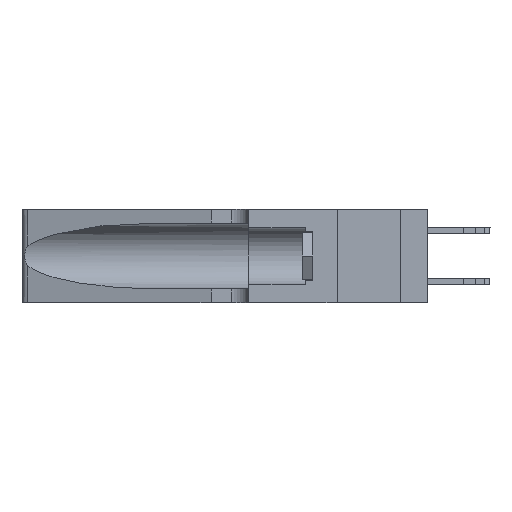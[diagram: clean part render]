
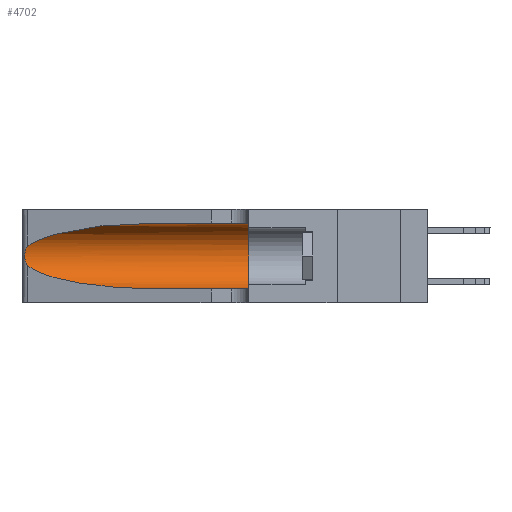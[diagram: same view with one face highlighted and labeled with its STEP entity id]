
A CAD part, left-side view. The second image highlights one B-rep face of the part: STEP entity #4702.
In plain terms, the highlighted cylindrical face has radius 3.308 mm (diameter 6.617 mm), a partial arc.
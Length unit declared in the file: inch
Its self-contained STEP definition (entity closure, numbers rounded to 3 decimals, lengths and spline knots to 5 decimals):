
#252 = CARTESIAN_POINT ( 'NONE',  ( 0.26018, 1.23835, 0.19895 ) ) ;
#362 = CARTESIAN_POINT ( 'NONE',  ( 0.25856, 1.23593, 0.16098 ) ) ;
#507 = CARTESIAN_POINT ( 'NONE',  ( 0.25487, 1.22718, 0.14631 ) ) ;
#692 = VERTEX_POINT ( 'NONE', #29806 ) ;
#1104 = ORIENTED_EDGE ( 'NONE', *, *, #36929, .T. ) ;
#3872 = CARTESIAN_POINT ( 'NONE',  ( 0.1305, 1.61858, 0.31525 ) ) ;
#4284 = CIRCLE ( 'NONE', #36613, 0.13025 ) ;
#4702 = ADVANCED_FACE ( 'NONE', ( #12334 ), #5035, .F. ) ;
#5035 = CYLINDRICAL_SURFACE ( 'NONE', #19683, 0.13025 ) ;
#5828 = DIRECTION ( 'NONE',  ( 0., -1., 0. ) ) ;
#6023 = CARTESIAN_POINT ( 'NONE',  ( 0.26075, 1.23896, 0.178 ) ) ;
#6257 = CARTESIAN_POINT ( 'NONE',  ( 0.25639, 1.23186, 0.15144 ) ) ;
#6469 = CARTESIAN_POINT ( 'NONE',  ( 0.1305, 1.61858, 0.05475 ) ) ;
#6514 = CARTESIAN_POINT ( 'NONE',  ( 0.25487, 1.22718, 0.22369 ) ) ;
#7052 =( BOUNDED_CURVE ( )  B_SPLINE_CURVE ( 3, ( #30509, #27434, #10241, #10376 ),
 .UNSPECIFIED., .F., .T. ) 
 B_SPLINE_CURVE_WITH_KNOTS ( ( 4, 4 ),
 ( 1.5708, 2.84003 ),
 .UNSPECIFIED. ) 
 CURVE ( )  GEOMETRIC_REPRESENTATION_ITEM ( )  RATIONAL_B_SPLINE_CURVE ( ( 1., 0.87, 0.87, 1. ) ) 
 REPRESENTATION_ITEM ( '' )  );
#7086 = ORIENTED_EDGE ( 'NONE', *, *, #24848, .T. ) ;
#7550 = CARTESIAN_POINT ( 'NONE',  ( 0.1305, 0.72297, 0.05475 ) ) ;
#9229 = CARTESIAN_POINT ( 'NONE',  ( 0.25555, 1.22993, 0.14849 ) ) ;
#9779 = VERTEX_POINT ( 'NONE', #31019 ) ;
#10241 = CARTESIAN_POINT ( 'NONE',  ( 0.2373, 1.15595, 0.28018 ) ) ;
#10376 = CARTESIAN_POINT ( 'NONE',  ( 0.25487, 1.22718, 0.22369 ) ) ;
#10410 = CARTESIAN_POINT ( 'NONE',  ( 0.18966, 0.96281, 0.05475 ) ) ;
#12138 = VERTEX_POINT ( 'NONE', #19780 ) ;
#12334 = FACE_OUTER_BOUND ( 'NONE', #36745, .T. ) ;
#12645 = LINE ( 'NONE', #6469, #25390 ) ;
#12689 = DIRECTION ( 'NONE',  ( 0., -1., 0. ) ) ;
#12705 = DIRECTION ( 'NONE',  ( 0., -1., 0. ) ) ;
#12967 = CARTESIAN_POINT ( 'NONE',  ( 0.1305, 1.61858, 0.185 ) ) ;
#13661 = DIRECTION ( 'NONE',  ( 0., 0., 1. ) ) ;
#15227 = CARTESIAN_POINT ( 'NONE',  ( 0.26017, 1.23833, 0.17102 ) ) ;
#15357 = CARTESIAN_POINT ( 'NONE',  ( 0.25787, 1.23484, 0.2124 ) ) ;
#15692 = CARTESIAN_POINT ( 'NONE',  ( 0.1305, 0.72297, 0.05475 ) ) ;
#15836 = VERTEX_POINT ( 'NONE', #34326 ) ;
#17000 = VECTOR ( 'NONE', #12705, 39.37008 ) ;
#17776 = CARTESIAN_POINT ( 'NONE',  ( 0.25555, 1.22994, 0.2215 ) ) ;
#17814 = B_SPLINE_CURVE_WITH_KNOTS ( 'NONE', 3,
 ( #6514, #17776, #29518, #15357, #23735, #252, #17895, #6023, #15227, #362, #20850, #6257, #9229, #507 ),
 .UNSPECIFIED., .F., .F.,
 ( 4, 2, 2, 2, 2, 2, 4 ),
 ( 0., 0.00027, 0.00053, 0.00107, 0.0016, 0.00187, 0.00214 ),
 .UNSPECIFIED. ) ;
#17895 = CARTESIAN_POINT ( 'NONE',  ( 0.26075, 1.23896, 0.19203 ) ) ;
#19333 = CARTESIAN_POINT ( 'NONE',  ( 0.2373, 1.15595, 0.08982 ) ) ;
#19367 = DIRECTION ( 'NONE',  ( 0., 1., 0. ) ) ;
#19499 =( BOUNDED_CURVE ( )  B_SPLINE_CURVE ( 3, ( #22374, #19333, #10410, #7550 ),
 .UNSPECIFIED., .F., .F. ) 
 B_SPLINE_CURVE_WITH_KNOTS ( ( 4, 4 ),
 ( 3.44316, 4.71239 ),
 .UNSPECIFIED. ) 
 CURVE ( )  GEOMETRIC_REPRESENTATION_ITEM ( )  RATIONAL_B_SPLINE_CURVE ( ( 1., 0.87, 0.87, 1. ) ) 
 REPRESENTATION_ITEM ( '' )  );
#19683 = AXIS2_PLACEMENT_3D ( 'NONE', #12967, #5828, #20038 ) ;
#19714 = ORIENTED_EDGE ( 'NONE', *, *, #20750, .F. ) ;
#19780 = CARTESIAN_POINT ( 'NONE',  ( 0.1305, 0.35, 0.31525 ) ) ;
#20038 = DIRECTION ( 'NONE',  ( 0., 0., -1. ) ) ;
#20750 = EDGE_CURVE ( 'NONE', #9779, #12138, #33421, .T. ) ;
#20850 = CARTESIAN_POINT ( 'NONE',  ( 0.25789, 1.23486, 0.15765 ) ) ;
#21015 = CARTESIAN_POINT ( 'NONE',  ( 0.25487, 1.22718, 0.14631 ) ) ;
#22374 = CARTESIAN_POINT ( 'NONE',  ( 0.25487, 1.22718, 0.14631 ) ) ;
#22917 = VERTEX_POINT ( 'NONE', #21015 ) ;
#23735 = CARTESIAN_POINT ( 'NONE',  ( 0.25854, 1.2359, 0.20912 ) ) ;
#24681 = EDGE_CURVE ( 'NONE', #35984, #692, #12645, .T. ) ;
#24848 = EDGE_CURVE ( 'NONE', #9779, #15836, #7052, .T. ) ;
#25390 = VECTOR ( 'NONE', #12689, 39.37008 ) ;
#27434 = CARTESIAN_POINT ( 'NONE',  ( 0.18966, 0.96281, 0.31525 ) ) ;
#28468 = EDGE_CURVE ( 'NONE', #12138, #692, #4284, .T. ) ;
#29518 = CARTESIAN_POINT ( 'NONE',  ( 0.25639, 1.23184, 0.21858 ) ) ;
#29806 = CARTESIAN_POINT ( 'NONE',  ( 0.1305, 0.35, 0.05475 ) ) ;
#30509 = CARTESIAN_POINT ( 'NONE',  ( 0.1305, 0.72297, 0.31525 ) ) ;
#31005 = ORIENTED_EDGE ( 'NONE', *, *, #37212, .T. ) ;
#31019 = CARTESIAN_POINT ( 'NONE',  ( 0.1305, 0.72297, 0.31525 ) ) ;
#33421 = LINE ( 'NONE', #3872, #17000 ) ;
#33894 = CARTESIAN_POINT ( 'NONE',  ( 0.1305, 0.35, 0.185 ) ) ;
#34326 = CARTESIAN_POINT ( 'NONE',  ( 0.25487, 1.22718, 0.22369 ) ) ;
#35496 = ORIENTED_EDGE ( 'NONE', *, *, #24681, .T. ) ;
#35522 = ORIENTED_EDGE ( 'NONE', *, *, #28468, .F. ) ;
#35984 = VERTEX_POINT ( 'NONE', #15692 ) ;
#36613 = AXIS2_PLACEMENT_3D ( 'NONE', #33894, #19367, #13661 ) ;
#36745 = EDGE_LOOP ( 'NONE', ( #7086, #1104, #31005, #35496, #35522, #19714 ) ) ;
#36929 = EDGE_CURVE ( 'NONE', #15836, #22917, #17814, .T. ) ;
#37212 = EDGE_CURVE ( 'NONE', #22917, #35984, #19499, .T. ) ;
